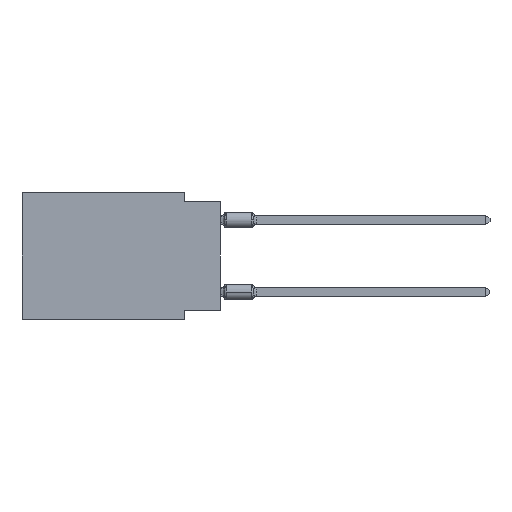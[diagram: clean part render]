
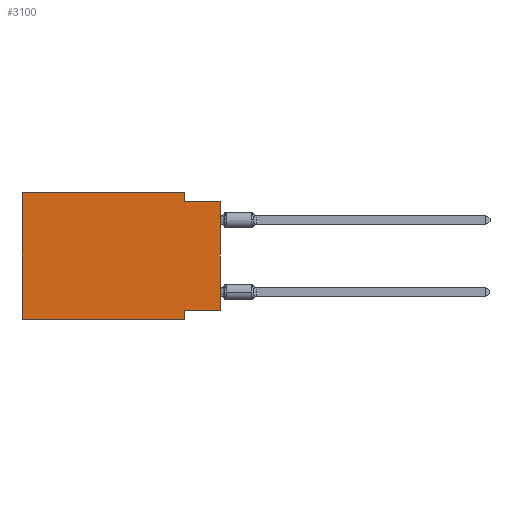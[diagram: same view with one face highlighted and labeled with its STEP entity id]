
A CAD part, left-side view. The second image highlights one B-rep face of the part: STEP entity #3100.
In plain terms, the highlighted planar face has unit normal (-1, 0, 0).
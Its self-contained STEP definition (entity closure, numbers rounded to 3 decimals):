
#169 = LINE ( 'NONE', #10508, #15824 ) ;
#723 = CARTESIAN_POINT ( 'NONE',  ( 0., 13.97, -8.89 ) ) ;
#953 = PLANE ( 'NONE',  #16024 ) ;
#1490 = CARTESIAN_POINT ( 'NONE',  ( 0., 13.97, 0. ) ) ;
#2150 = DIRECTION ( 'NONE',  ( 0., -1., 0. ) ) ;
#2287 = EDGE_CURVE ( 'NONE', #13660, #10430, #13033, .T. ) ;
#2605 = ORIENTED_EDGE ( 'NONE', *, *, #6178, .T. ) ;
#2847 = LINE ( 'NONE', #1490, #6646 ) ;
#2877 = CARTESIAN_POINT ( 'NONE',  ( 0., 13.97, 0. ) ) ;
#3100 = ADVANCED_FACE ( 'NONE', ( #12548 ), #953, .F. ) ;
#3488 = DIRECTION ( 'NONE',  ( 0., 0., -1. ) ) ;
#3637 = EDGE_CURVE ( 'NONE', #16363, #13660, #169, .T. ) ;
#4211 = ORIENTED_EDGE ( 'NONE', *, *, #9218, .F. ) ;
#4231 = DIRECTION ( 'NONE',  ( 0., 0., -1. ) ) ;
#4902 = LINE ( 'NONE', #8704, #10829 ) ;
#5130 = CARTESIAN_POINT ( 'NONE',  ( 0., 0., -0.635 ) ) ;
#5382 = EDGE_CURVE ( 'NONE', #6639, #16629, #4902, .T. ) ;
#5548 = DIRECTION ( 'NONE',  ( 0., 0., 1. ) ) ;
#6096 = VECTOR ( 'NONE', #15492, 1000. ) ;
#6178 = EDGE_CURVE ( 'NONE', #10910, #7180, #16136, .T. ) ;
#6639 = VERTEX_POINT ( 'NONE', #15349 ) ;
#6646 = VECTOR ( 'NONE', #5548, 1000. ) ;
#6649 = ORIENTED_EDGE ( 'NONE', *, *, #3637, .F. ) ;
#6774 = DIRECTION ( 'NONE',  ( 0., -1., 0. ) ) ;
#7179 = CARTESIAN_POINT ( 'NONE',  ( 0., 2.54, -8.89 ) ) ;
#7180 = VERTEX_POINT ( 'NONE', #11994 ) ;
#7332 = LINE ( 'NONE', #12497, #12317 ) ;
#7627 = ORIENTED_EDGE ( 'NONE', *, *, #14287, .F. ) ;
#8614 = CARTESIAN_POINT ( 'NONE',  ( 0., 2.54, -8.255 ) ) ;
#8704 = CARTESIAN_POINT ( 'NONE',  ( 0., 0., -8.255 ) ) ;
#9030 = EDGE_CURVE ( 'NONE', #6639, #10430, #7332, .T. ) ;
#9218 = EDGE_CURVE ( 'NONE', #10910, #10765, #2847, .T. ) ;
#9552 = LINE ( 'NONE', #7179, #16375 ) ;
#10034 = VECTOR ( 'NONE', #2150, 1000. ) ;
#10097 = CARTESIAN_POINT ( 'NONE',  ( 0., 13.97, 0. ) ) ;
#10181 = ORIENTED_EDGE ( 'NONE', *, *, #5382, .F. ) ;
#10430 = VERTEX_POINT ( 'NONE', #5130 ) ;
#10508 = CARTESIAN_POINT ( 'NONE',  ( 0., 2.54, 0. ) ) ;
#10765 = VERTEX_POINT ( 'NONE', #10097 ) ;
#10829 = VECTOR ( 'NONE', #16418, 1000. ) ;
#10910 = VERTEX_POINT ( 'NONE', #13569 ) ;
#11136 = EDGE_LOOP ( 'NONE', ( #12593, #11695, #6649, #7627, #4211, #2605, #14739, #10181 ) ) ;
#11317 = DIRECTION ( 'NONE',  ( 0., 0., 1. ) ) ;
#11431 = DIRECTION ( 'NONE',  ( 0., 0., -1. ) ) ;
#11448 = VECTOR ( 'NONE', #6774, 1000. ) ;
#11695 = ORIENTED_EDGE ( 'NONE', *, *, #2287, .F. ) ;
#11994 = CARTESIAN_POINT ( 'NONE',  ( 0., 2.54, -8.89 ) ) ;
#12015 = LINE ( 'NONE', #2877, #11448 ) ;
#12317 = VECTOR ( 'NONE', #11317, 1000. ) ;
#12497 = CARTESIAN_POINT ( 'NONE',  ( 0., 0., 0. ) ) ;
#12548 = FACE_OUTER_BOUND ( 'NONE', #11136, .T. ) ;
#12593 = ORIENTED_EDGE ( 'NONE', *, *, #9030, .T. ) ;
#12641 = CARTESIAN_POINT ( 'NONE',  ( 0., 13.97, 0. ) ) ;
#12779 = CARTESIAN_POINT ( 'NONE',  ( 0., 0., -0.635 ) ) ;
#13033 = LINE ( 'NONE', #12779, #6096 ) ;
#13569 = CARTESIAN_POINT ( 'NONE',  ( 0., 13.97, -8.89 ) ) ;
#13660 = VERTEX_POINT ( 'NONE', #15118 ) ;
#14287 = EDGE_CURVE ( 'NONE', #10765, #16363, #12015, .T. ) ;
#14739 = ORIENTED_EDGE ( 'NONE', *, *, #16495, .F. ) ;
#15097 = DIRECTION ( 'NONE',  ( 1., 0., 0. ) ) ;
#15118 = CARTESIAN_POINT ( 'NONE',  ( 0., 2.54, -0.635 ) ) ;
#15253 = CARTESIAN_POINT ( 'NONE',  ( 0., 2.54, 0. ) ) ;
#15349 = CARTESIAN_POINT ( 'NONE',  ( 0., 0., -8.255 ) ) ;
#15492 = DIRECTION ( 'NONE',  ( 0., -1., 0. ) ) ;
#15824 = VECTOR ( 'NONE', #11431, 1000. ) ;
#16024 = AXIS2_PLACEMENT_3D ( 'NONE', #12641, #15097, #3488 ) ;
#16136 = LINE ( 'NONE', #723, #10034 ) ;
#16363 = VERTEX_POINT ( 'NONE', #15253 ) ;
#16375 = VECTOR ( 'NONE', #4231, 1000. ) ;
#16418 = DIRECTION ( 'NONE',  ( 0., 1., 0. ) ) ;
#16495 = EDGE_CURVE ( 'NONE', #16629, #7180, #9552, .T. ) ;
#16629 = VERTEX_POINT ( 'NONE', #8614 ) ;
